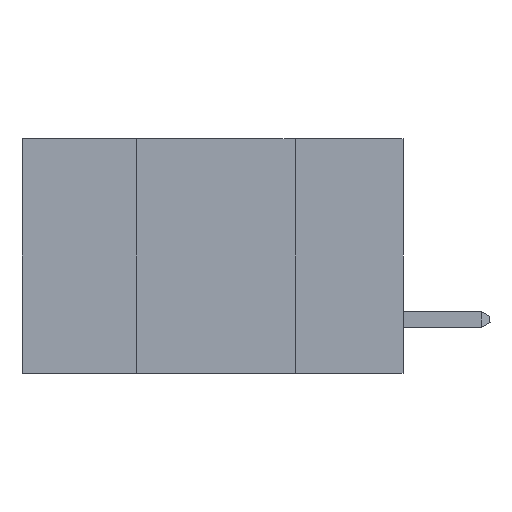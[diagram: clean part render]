
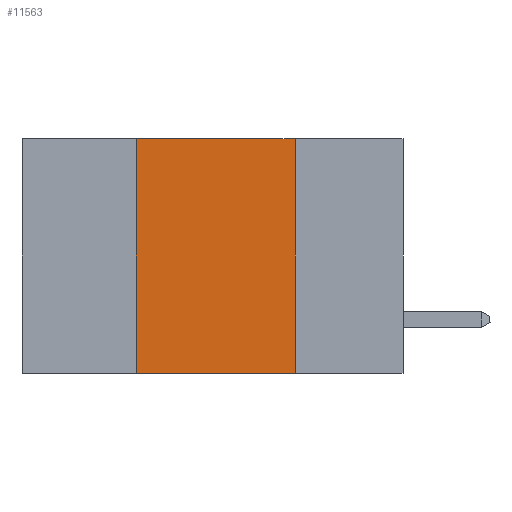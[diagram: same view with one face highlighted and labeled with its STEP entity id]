
A CAD part, left-side view. The second image highlights one B-rep face of the part: STEP entity #11563.
In plain terms, the highlighted planar face has unit normal (-1, 0, 0).
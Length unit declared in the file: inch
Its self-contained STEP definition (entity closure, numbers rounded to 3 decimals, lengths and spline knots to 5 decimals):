
#753 = CARTESIAN_POINT ( 'NONE',  ( 0., 0.42, -0.37 ) ) ;
#1363 = CARTESIAN_POINT ( 'NONE',  ( 0., 0.6, -0.37 ) ) ;
#1628 = CARTESIAN_POINT ( 'NONE',  ( 0., 0.6, 0. ) ) ;
#1924 = LINE ( 'NONE', #10304, #19118 ) ;
#2489 = FACE_OUTER_BOUND ( 'NONE', #18263, .T. ) ;
#2686 = CARTESIAN_POINT ( 'NONE',  ( 0., 0.42, 0. ) ) ;
#3127 = DIRECTION ( 'NONE',  ( 0., -1., 0. ) ) ;
#3429 = DIRECTION ( 'NONE',  ( 1., 0., 0. ) ) ;
#3677 = LINE ( 'NONE', #2686, #19680 ) ;
#5792 = VECTOR ( 'NONE', #7836, 39.37008 ) ;
#7523 = ORIENTED_EDGE ( 'NONE', *, *, #19089, .F. ) ;
#7836 = DIRECTION ( 'NONE',  ( 0., 0., -1. ) ) ;
#8652 = LINE ( 'NONE', #1363, #15254 ) ;
#9984 = ORIENTED_EDGE ( 'NONE', *, *, #20536, .F. ) ;
#10304 = CARTESIAN_POINT ( 'NONE',  ( 0., 0.6, 0. ) ) ;
#11563 = ADVANCED_FACE ( 'NONE', ( #2489 ), #21783, .F. ) ;
#12444 = VERTEX_POINT ( 'NONE', #14165 ) ;
#12669 = DIRECTION ( 'NONE',  ( 0., 0., -1. ) ) ;
#13009 = CARTESIAN_POINT ( 'NONE',  ( 0., 0.17, 0. ) ) ;
#13268 = AXIS2_PLACEMENT_3D ( 'NONE', #1628, #3429, #12669 ) ;
#13796 = VERTEX_POINT ( 'NONE', #13009 ) ;
#14165 = CARTESIAN_POINT ( 'NONE',  ( 0., 0.42, 0. ) ) ;
#15207 = VERTEX_POINT ( 'NONE', #18181 ) ;
#15254 = VECTOR ( 'NONE', #16157, 39.37008 ) ;
#16157 = DIRECTION ( 'NONE',  ( 0., -1., 0. ) ) ;
#16342 = ORIENTED_EDGE ( 'NONE', *, *, #20601, .F. ) ;
#18181 = CARTESIAN_POINT ( 'NONE',  ( 0., 0.17, -0.37 ) ) ;
#18263 = EDGE_LOOP ( 'NONE', ( #7523, #9984, #16342, #22214 ) ) ;
#18918 = DIRECTION ( 'NONE',  ( 0., 0., 1. ) ) ;
#19089 = EDGE_CURVE ( 'NONE', #13796, #15207, #19836, .T. ) ;
#19118 = VECTOR ( 'NONE', #3127, 39.37008 ) ;
#19584 = VERTEX_POINT ( 'NONE', #753 ) ;
#19680 = VECTOR ( 'NONE', #18918, 39.37008 ) ;
#19836 = LINE ( 'NONE', #20381, #5792 ) ;
#20381 = CARTESIAN_POINT ( 'NONE',  ( 0., 0.17, 0. ) ) ;
#20536 = EDGE_CURVE ( 'NONE', #12444, #13796, #1924, .T. ) ;
#20601 = EDGE_CURVE ( 'NONE', #19584, #12444, #3677, .T. ) ;
#21783 = PLANE ( 'NONE',  #13268 ) ;
#22214 = ORIENTED_EDGE ( 'NONE', *, *, #23441, .T. ) ;
#23441 = EDGE_CURVE ( 'NONE', #19584, #15207, #8652, .T. ) ;
